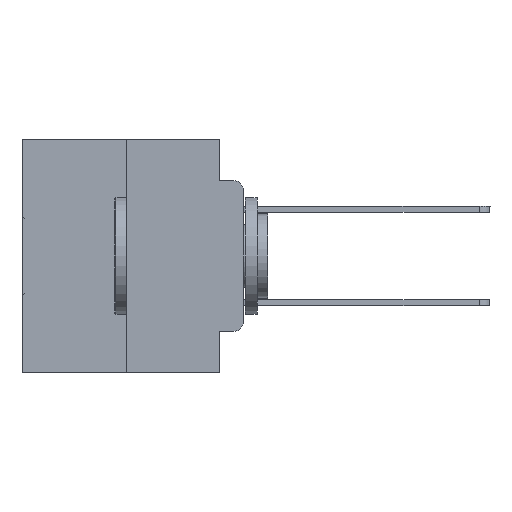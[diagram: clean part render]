
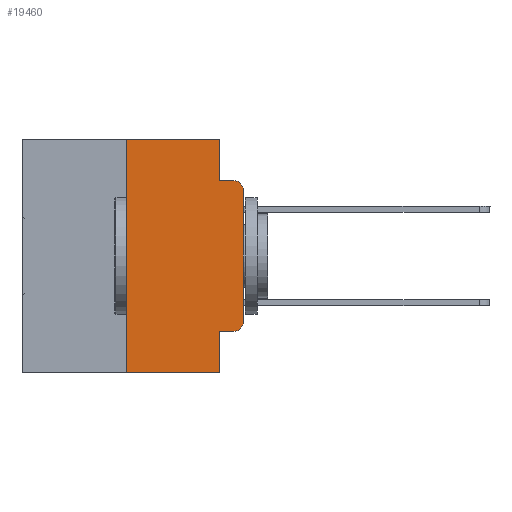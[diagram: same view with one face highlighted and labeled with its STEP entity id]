
A CAD part, left-side view. The second image highlights one B-rep face of the part: STEP entity #19460.
In plain terms, the highlighted planar face has unit normal (-1, 0, 0).
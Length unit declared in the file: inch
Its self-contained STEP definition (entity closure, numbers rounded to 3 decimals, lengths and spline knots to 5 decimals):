
#587 = CARTESIAN_POINT ( 'NONE',  ( 0., 0.051, -0.0885 ) ) ;
#980 = EDGE_CURVE ( 'NONE', #12237, #18086, #1984, .T. ) ;
#1299 = LINE ( 'NONE', #4189, #13982 ) ;
#1328 = DIRECTION ( 'NONE',  ( 0., 0., -1. ) ) ;
#1424 = CARTESIAN_POINT ( 'NONE',  ( 0., 0.051, -0.4115 ) ) ;
#1548 = AXIS2_PLACEMENT_3D ( 'NONE', #15651, #3092, #25806 ) ;
#1640 = DIRECTION ( 'NONE',  ( 0., -1., 0. ) ) ;
#1984 = LINE ( 'NONE', #32558, #29296 ) ;
#2610 = AXIS2_PLACEMENT_3D ( 'NONE', #7050, #17249, #6571 ) ;
#3092 = DIRECTION ( 'NONE',  ( -1., 0., 0. ) ) ;
#3206 = CARTESIAN_POINT ( 'NONE',  ( 0., 0., -0.3915 ) ) ;
#3705 = ORIENTED_EDGE ( 'NONE', *, *, #14567, .F. ) ;
#3745 = VERTEX_POINT ( 'NONE', #5296 ) ;
#4181 = LINE ( 'NONE', #19542, #26449 ) ;
#4189 = CARTESIAN_POINT ( 'NONE',  ( 0., 0.473, -0.5 ) ) ;
#4363 = DIRECTION ( 'NONE',  ( 0., -1., 0. ) ) ;
#4968 = ORIENTED_EDGE ( 'NONE', *, *, #980, .F. ) ;
#5004 = VERTEX_POINT ( 'NONE', #16869 ) ;
#5296 = CARTESIAN_POINT ( 'NONE',  ( 0., 0., -0.1085 ) ) ;
#5577 = EDGE_CURVE ( 'NONE', #27179, #8828, #10970, .T. ) ;
#5767 = DIRECTION ( 'NONE',  ( 0., -1., 0. ) ) ;
#6339 = VERTEX_POINT ( 'NONE', #11163 ) ;
#6571 = DIRECTION ( 'NONE',  ( 0., 0., -1. ) ) ;
#6704 = ORIENTED_EDGE ( 'NONE', *, *, #11401, .T. ) ;
#7050 = CARTESIAN_POINT ( 'NONE',  ( 0., 0.473, 0. ) ) ;
#7546 = DIRECTION ( 'NONE',  ( 0., 0., 1. ) ) ;
#7794 = VECTOR ( 'NONE', #20307, 39.37008 ) ;
#8583 = EDGE_CURVE ( 'NONE', #27179, #18823, #12635, .T. ) ;
#8828 = VERTEX_POINT ( 'NONE', #16946 ) ;
#8950 = CIRCLE ( 'NONE', #18000, 0.02 ) ;
#9234 = FACE_OUTER_BOUND ( 'NONE', #22536, .T. ) ;
#9837 = VECTOR ( 'NONE', #7546, 39.37008 ) ;
#10376 = ORIENTED_EDGE ( 'NONE', *, *, #20147, .T. ) ;
#10970 = LINE ( 'NONE', #15802, #23708 ) ;
#11163 = CARTESIAN_POINT ( 'NONE',  ( 0., 0.051, 0. ) ) ;
#11401 = EDGE_CURVE ( 'NONE', #8828, #31410, #8950, .T. ) ;
#12237 = VERTEX_POINT ( 'NONE', #587 ) ;
#12635 = LINE ( 'NONE', #30150, #7794 ) ;
#12694 = ORIENTED_EDGE ( 'NONE', *, *, #25258, .T. ) ;
#12865 = EDGE_CURVE ( 'NONE', #5004, #30914, #30412, .T. ) ;
#12891 = DIRECTION ( 'NONE',  ( 0., 0., 1. ) ) ;
#13815 = ORIENTED_EDGE ( 'NONE', *, *, #22538, .T. ) ;
#13982 = VECTOR ( 'NONE', #1640, 39.37008 ) ;
#14243 = CARTESIAN_POINT ( 'NONE',  ( 0., 0.051, -0.5 ) ) ;
#14567 = EDGE_CURVE ( 'NONE', #30914, #6339, #24888, .T. ) ;
#15651 = CARTESIAN_POINT ( 'NONE',  ( 0., 0.02, -0.1085 ) ) ;
#15802 = CARTESIAN_POINT ( 'NONE',  ( 0., 0.051, -0.4115 ) ) ;
#16869 = CARTESIAN_POINT ( 'NONE',  ( 0., 0.25, -0.5 ) ) ;
#16876 = DIRECTION ( 'NONE',  ( 0., 0., -1. ) ) ;
#16946 = CARTESIAN_POINT ( 'NONE',  ( 0., 0.02, -0.4115 ) ) ;
#17022 = ORIENTED_EDGE ( 'NONE', *, *, #12865, .F. ) ;
#17249 = DIRECTION ( 'NONE',  ( 1., 0., 0. ) ) ;
#17725 = LINE ( 'NONE', #22926, #26985 ) ;
#18000 = AXIS2_PLACEMENT_3D ( 'NONE', #18754, #21437, #1328 ) ;
#18086 = VERTEX_POINT ( 'NONE', #20822 ) ;
#18754 = CARTESIAN_POINT ( 'NONE',  ( 0., 0.02, -0.3915 ) ) ;
#18823 = VERTEX_POINT ( 'NONE', #14243 ) ;
#19460 = ADVANCED_FACE ( 'NONE', ( #9234 ), #29591, .F. ) ;
#19542 = CARTESIAN_POINT ( 'NONE',  ( 0., 0.051, 0. ) ) ;
#19554 = CARTESIAN_POINT ( 'NONE',  ( 0., 0.473, 0. ) ) ;
#20147 = EDGE_CURVE ( 'NONE', #3745, #18086, #30917, .T. ) ;
#20307 = DIRECTION ( 'NONE',  ( 0., 0., -1. ) ) ;
#20822 = CARTESIAN_POINT ( 'NONE',  ( 0., 0.02, -0.0885 ) ) ;
#21437 = DIRECTION ( 'NONE',  ( -1., 0., 0. ) ) ;
#22536 = EDGE_LOOP ( 'NONE', ( #12694, #10376, #4968, #32416, #3705, #17022, #13815, #26103, #23920, #6704 ) ) ;
#22538 = EDGE_CURVE ( 'NONE', #5004, #18823, #1299, .T. ) ;
#22926 = CARTESIAN_POINT ( 'NONE',  ( 0., 0., 0. ) ) ;
#23708 = VECTOR ( 'NONE', #5767, 39.37008 ) ;
#23920 = ORIENTED_EDGE ( 'NONE', *, *, #5577, .T. ) ;
#24888 = LINE ( 'NONE', #19554, #27493 ) ;
#25258 = EDGE_CURVE ( 'NONE', #31410, #3745, #17725, .T. ) ;
#25409 = EDGE_CURVE ( 'NONE', #6339, #12237, #4181, .T. ) ;
#25806 = DIRECTION ( 'NONE',  ( 0., 0., -1. ) ) ;
#26103 = ORIENTED_EDGE ( 'NONE', *, *, #8583, .F. ) ;
#26449 = VECTOR ( 'NONE', #16876, 39.37008 ) ;
#26985 = VECTOR ( 'NONE', #12891, 39.37008 ) ;
#27179 = VERTEX_POINT ( 'NONE', #1424 ) ;
#27493 = VECTOR ( 'NONE', #30382, 39.37008 ) ;
#27565 = CARTESIAN_POINT ( 'NONE',  ( 0., 0.25, 0. ) ) ;
#29296 = VECTOR ( 'NONE', #4363, 39.37008 ) ;
#29591 = PLANE ( 'NONE',  #2610 ) ;
#30150 = CARTESIAN_POINT ( 'NONE',  ( 0., 0.051, 0. ) ) ;
#30382 = DIRECTION ( 'NONE',  ( 0., -1., 0. ) ) ;
#30412 = LINE ( 'NONE', #27565, #9837 ) ;
#30914 = VERTEX_POINT ( 'NONE', #31300 ) ;
#30917 = CIRCLE ( 'NONE', #1548, 0.02 ) ;
#31300 = CARTESIAN_POINT ( 'NONE',  ( 0., 0.25, 0. ) ) ;
#31410 = VERTEX_POINT ( 'NONE', #3206 ) ;
#32416 = ORIENTED_EDGE ( 'NONE', *, *, #25409, .F. ) ;
#32558 = CARTESIAN_POINT ( 'NONE',  ( 0., 0.051, -0.0885 ) ) ;
